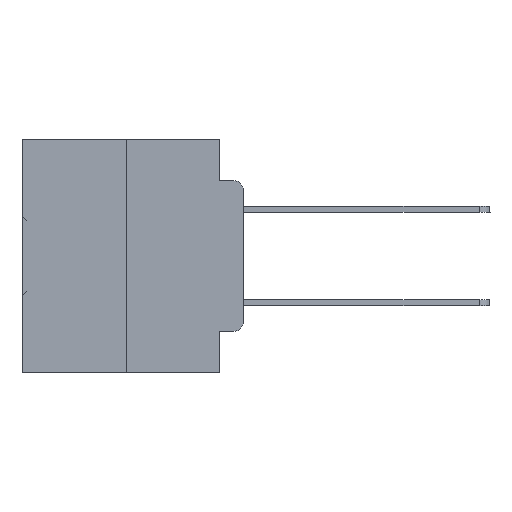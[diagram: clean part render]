
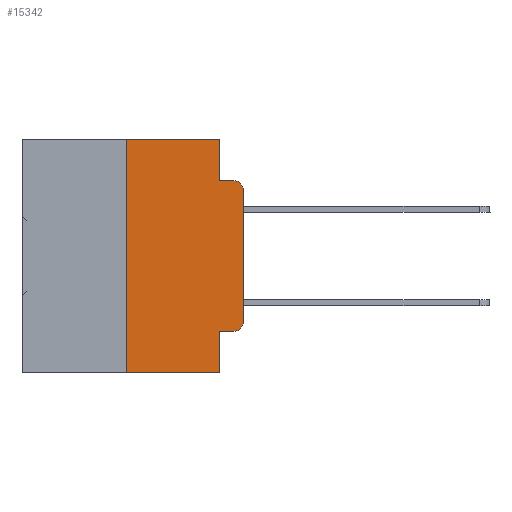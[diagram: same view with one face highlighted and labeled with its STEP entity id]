
A CAD part, left-side view. The second image highlights one B-rep face of the part: STEP entity #15342.
In plain terms, the highlighted planar face has unit normal (-1, 0, 0).
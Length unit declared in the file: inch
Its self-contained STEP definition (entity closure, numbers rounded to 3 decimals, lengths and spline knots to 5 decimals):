
#289 = DIRECTION ( 'NONE',  ( -1., 0., 0. ) ) ;
#413 = AXIS2_PLACEMENT_3D ( 'NONE', #25657, #30919, #8291 ) ;
#1415 = VERTEX_POINT ( 'NONE', #31669 ) ;
#1441 = CARTESIAN_POINT ( 'NONE',  ( 0., 0., 0. ) ) ;
#1775 = VERTEX_POINT ( 'NONE', #12298 ) ;
#2214 = DIRECTION ( 'NONE',  ( 0., -1., 0. ) ) ;
#2299 = CARTESIAN_POINT ( 'NONE',  ( 0., 0.02, -0.0885 ) ) ;
#2362 = EDGE_CURVE ( 'NONE', #1775, #3293, #16693, .T. ) ;
#2689 = LINE ( 'NONE', #13020, #31562 ) ;
#2786 = CIRCLE ( 'NONE', #26665, 0.02 ) ;
#3293 = VERTEX_POINT ( 'NONE', #2299 ) ;
#3815 = ORIENTED_EDGE ( 'NONE', *, *, #33207, .F. ) ;
#4537 = VECTOR ( 'NONE', #31582, 39.37008 ) ;
#5068 = VERTEX_POINT ( 'NONE', #25862 ) ;
#5770 = CARTESIAN_POINT ( 'NONE',  ( 0., 0.051, 0. ) ) ;
#5856 = FACE_OUTER_BOUND ( 'NONE', #35678, .T. ) ;
#5956 = CARTESIAN_POINT ( 'NONE',  ( 0., 0.25, 0. ) ) ;
#6628 = LINE ( 'NONE', #1441, #32332 ) ;
#6783 = VECTOR ( 'NONE', #19901, 39.37008 ) ;
#7196 = VECTOR ( 'NONE', #21290, 39.37008 ) ;
#8012 = EDGE_CURVE ( 'NONE', #1415, #34596, #25362, .T. ) ;
#8291 = DIRECTION ( 'NONE',  ( 0., 0., -1. ) ) ;
#9116 = EDGE_CURVE ( 'NONE', #10507, #16192, #2689, .T. ) ;
#10431 = PLANE ( 'NONE',  #36429 ) ;
#10507 = VERTEX_POINT ( 'NONE', #21356 ) ;
#10687 = CARTESIAN_POINT ( 'NONE',  ( 0., 0.473, 0. ) ) ;
#10803 = ORIENTED_EDGE ( 'NONE', *, *, #11085, .F. ) ;
#11085 = EDGE_CURVE ( 'NONE', #5068, #1775, #11969, .T. ) ;
#11969 = LINE ( 'NONE', #5770, #29619 ) ;
#12298 = CARTESIAN_POINT ( 'NONE',  ( 0., 0.051, -0.0885 ) ) ;
#12963 = VECTOR ( 'NONE', #35684, 39.37008 ) ;
#13020 = CARTESIAN_POINT ( 'NONE',  ( 0., 0.051, -0.4115 ) ) ;
#13155 = EDGE_CURVE ( 'NONE', #33670, #31463, #6628, .T. ) ;
#13399 = VERTEX_POINT ( 'NONE', #17169 ) ;
#13603 = DIRECTION ( 'NONE',  ( 0., 0., -1. ) ) ;
#14147 = CARTESIAN_POINT ( 'NONE',  ( 0., 0.25, 0. ) ) ;
#14449 = LINE ( 'NONE', #17073, #6783 ) ;
#14926 = ORIENTED_EDGE ( 'NONE', *, *, #9116, .T. ) ;
#15342 = ADVANCED_FACE ( 'NONE', ( #5856 ), #10431, .F. ) ;
#16192 = VERTEX_POINT ( 'NONE', #20028 ) ;
#16693 = LINE ( 'NONE', #24081, #7196 ) ;
#17073 = CARTESIAN_POINT ( 'NONE',  ( 0., 0.473, 0. ) ) ;
#17169 = CARTESIAN_POINT ( 'NONE',  ( 0., 0.051, -0.5 ) ) ;
#18029 = DIRECTION ( 'NONE',  ( 0., 0., -1. ) ) ;
#18229 = ORIENTED_EDGE ( 'NONE', *, *, #2362, .F. ) ;
#18287 = CARTESIAN_POINT ( 'NONE',  ( 0., 0.051, 0. ) ) ;
#18604 = DIRECTION ( 'NONE',  ( 0., 0., 1. ) ) ;
#19862 = CARTESIAN_POINT ( 'NONE',  ( 0., 0.02, -0.1085 ) ) ;
#19901 = DIRECTION ( 'NONE',  ( 0., -1., 0. ) ) ;
#20028 = CARTESIAN_POINT ( 'NONE',  ( 0., 0.02, -0.4115 ) ) ;
#21290 = DIRECTION ( 'NONE',  ( 0., -1., 0. ) ) ;
#21356 = CARTESIAN_POINT ( 'NONE',  ( 0., 0.051, -0.4115 ) ) ;
#21982 = LINE ( 'NONE', #32055, #25150 ) ;
#22088 = ORIENTED_EDGE ( 'NONE', *, *, #13155, .T. ) ;
#23616 = DIRECTION ( 'NONE',  ( 0., -1., 0. ) ) ;
#23761 = EDGE_CURVE ( 'NONE', #34596, #5068, #14449, .T. ) ;
#24081 = CARTESIAN_POINT ( 'NONE',  ( 0., 0.051, -0.0885 ) ) ;
#24577 = CIRCLE ( 'NONE', #413, 0.02 ) ;
#25150 = VECTOR ( 'NONE', #23616, 39.37008 ) ;
#25362 = LINE ( 'NONE', #5956, #4537 ) ;
#25657 = CARTESIAN_POINT ( 'NONE',  ( 0., 0.02, -0.3915 ) ) ;
#25862 = CARTESIAN_POINT ( 'NONE',  ( 0., 0.051, 0. ) ) ;
#25977 = DIRECTION ( 'NONE',  ( 0., 0., -1. ) ) ;
#26040 = EDGE_CURVE ( 'NONE', #31463, #3293, #2786, .T. ) ;
#26665 = AXIS2_PLACEMENT_3D ( 'NONE', #19862, #289, #18029 ) ;
#27516 = ORIENTED_EDGE ( 'NONE', *, *, #23761, .F. ) ;
#27740 = ORIENTED_EDGE ( 'NONE', *, *, #8012, .F. ) ;
#27906 = DIRECTION ( 'NONE',  ( 1., 0., 0. ) ) ;
#29412 = EDGE_CURVE ( 'NONE', #1415, #13399, #21982, .T. ) ;
#29596 = CARTESIAN_POINT ( 'NONE',  ( 0., 0., -0.3915 ) ) ;
#29619 = VECTOR ( 'NONE', #25977, 39.37008 ) ;
#30919 = DIRECTION ( 'NONE',  ( -1., 0., 0. ) ) ;
#31463 = VERTEX_POINT ( 'NONE', #34648 ) ;
#31562 = VECTOR ( 'NONE', #2214, 39.37008 ) ;
#31582 = DIRECTION ( 'NONE',  ( 0., 0., 1. ) ) ;
#31669 = CARTESIAN_POINT ( 'NONE',  ( 0., 0.25, -0.5 ) ) ;
#32055 = CARTESIAN_POINT ( 'NONE',  ( 0., 0.473, -0.5 ) ) ;
#32332 = VECTOR ( 'NONE', #18604, 39.37008 ) ;
#33207 = EDGE_CURVE ( 'NONE', #10507, #13399, #33743, .T. ) ;
#33670 = VERTEX_POINT ( 'NONE', #29596 ) ;
#33743 = LINE ( 'NONE', #18287, #12963 ) ;
#34596 = VERTEX_POINT ( 'NONE', #14147 ) ;
#34648 = CARTESIAN_POINT ( 'NONE',  ( 0., 0., -0.1085 ) ) ;
#34887 = ORIENTED_EDGE ( 'NONE', *, *, #35117, .T. ) ;
#35117 = EDGE_CURVE ( 'NONE', #16192, #33670, #24577, .T. ) ;
#35678 = EDGE_LOOP ( 'NONE', ( #22088, #36956, #18229, #10803, #27516, #27740, #36241, #3815, #14926, #34887 ) ) ;
#35684 = DIRECTION ( 'NONE',  ( 0., 0., -1. ) ) ;
#36241 = ORIENTED_EDGE ( 'NONE', *, *, #29412, .T. ) ;
#36429 = AXIS2_PLACEMENT_3D ( 'NONE', #10687, #27906, #13603 ) ;
#36956 = ORIENTED_EDGE ( 'NONE', *, *, #26040, .T. ) ;
